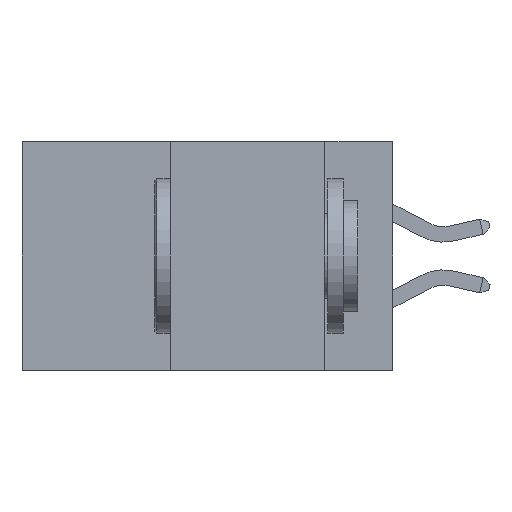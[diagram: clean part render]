
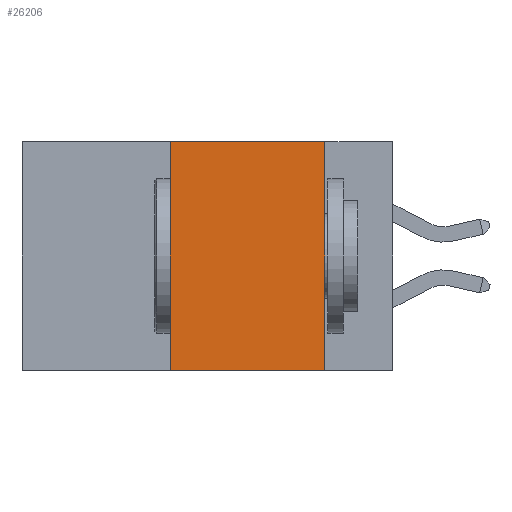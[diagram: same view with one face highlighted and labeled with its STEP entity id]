
A CAD part, left-side view. The second image highlights one B-rep face of the part: STEP entity #26206.
In plain terms, the highlighted planar face has unit normal (-1, 0, 0).
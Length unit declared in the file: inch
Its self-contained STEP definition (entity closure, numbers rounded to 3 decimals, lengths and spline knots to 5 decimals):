
#891 = EDGE_CURVE ( 'NONE', #2135, #4056, #29113, .T. ) ;
#1875 = CARTESIAN_POINT ( 'NONE',  ( 0., 0.11, 0. ) ) ;
#2135 = VERTEX_POINT ( 'NONE', #3306 ) ;
#3306 = CARTESIAN_POINT ( 'NONE',  ( 0., 0.36, 0. ) ) ;
#3590 = AXIS2_PLACEMENT_3D ( 'NONE', #41190, #22111, #41479 ) ;
#3888 = ORIENTED_EDGE ( 'NONE', *, *, #15936, .T. ) ;
#4056 = VERTEX_POINT ( 'NONE', #1875 ) ;
#4066 = DIRECTION ( 'NONE',  ( 0., 0., -1. ) ) ;
#4876 = VECTOR ( 'NONE', #4066, 39.37008 ) ;
#7153 = CARTESIAN_POINT ( 'NONE',  ( 0., 0.36, -0.37 ) ) ;
#7158 = EDGE_LOOP ( 'NONE', ( #15432, #14532, #39005, #3888 ) ) ;
#7579 = CARTESIAN_POINT ( 'NONE',  ( 0., 0.11, 0. ) ) ;
#7878 = LINE ( 'NONE', #35758, #15429 ) ;
#8935 = CARTESIAN_POINT ( 'NONE',  ( 0., 0.6, 0. ) ) ;
#9513 = CARTESIAN_POINT ( 'NONE',  ( 0., 0.6, -0.37 ) ) ;
#13784 = CARTESIAN_POINT ( 'NONE',  ( 0., 0.11, -0.37 ) ) ;
#14532 = ORIENTED_EDGE ( 'NONE', *, *, #891, .F. ) ;
#15403 = DIRECTION ( 'NONE',  ( 0., -1., 0. ) ) ;
#15429 = VECTOR ( 'NONE', #16439, 39.37008 ) ;
#15432 = ORIENTED_EDGE ( 'NONE', *, *, #15564, .F. ) ;
#15564 = EDGE_CURVE ( 'NONE', #4056, #15610, #33114, .T. ) ;
#15610 = VERTEX_POINT ( 'NONE', #13784 ) ;
#15936 = EDGE_CURVE ( 'NONE', #30950, #15610, #40164, .T. ) ;
#16439 = DIRECTION ( 'NONE',  ( 0., 0., 1. ) ) ;
#18590 = PLANE ( 'NONE',  #3590 ) ;
#19457 = VECTOR ( 'NONE', #22326, 39.37008 ) ;
#22111 = DIRECTION ( 'NONE',  ( 1., 0., 0. ) ) ;
#22326 = DIRECTION ( 'NONE',  ( 0., -1., 0. ) ) ;
#26040 = FACE_OUTER_BOUND ( 'NONE', #7158, .T. ) ;
#26206 = ADVANCED_FACE ( 'NONE', ( #26040 ), #18590, .F. ) ;
#29113 = LINE ( 'NONE', #8935, #33672 ) ;
#30950 = VERTEX_POINT ( 'NONE', #7153 ) ;
#32792 = EDGE_CURVE ( 'NONE', #30950, #2135, #7878, .T. ) ;
#33114 = LINE ( 'NONE', #7579, #4876 ) ;
#33672 = VECTOR ( 'NONE', #15403, 39.37008 ) ;
#35758 = CARTESIAN_POINT ( 'NONE',  ( 0., 0.36, 0. ) ) ;
#39005 = ORIENTED_EDGE ( 'NONE', *, *, #32792, .F. ) ;
#40164 = LINE ( 'NONE', #9513, #19457 ) ;
#41190 = CARTESIAN_POINT ( 'NONE',  ( 0., 0.6, 0. ) ) ;
#41479 = DIRECTION ( 'NONE',  ( 0., 0., -1. ) ) ;
